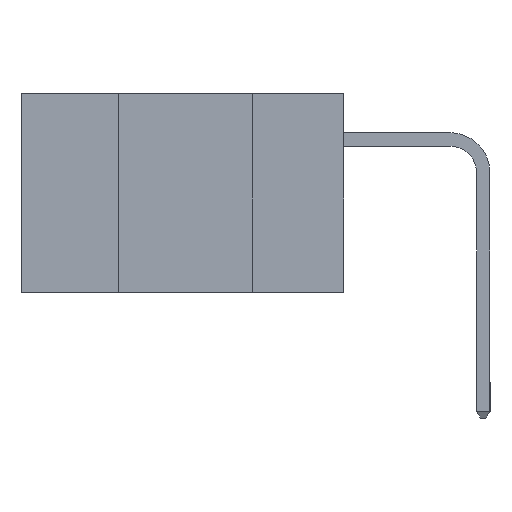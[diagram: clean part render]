
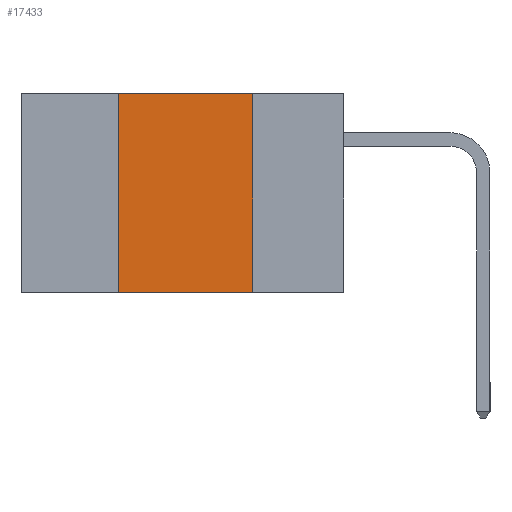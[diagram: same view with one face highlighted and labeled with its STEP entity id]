
A CAD part, left-side view. The second image highlights one B-rep face of the part: STEP entity #17433.
In plain terms, the highlighted planar face has unit normal (-1, 0, 0).
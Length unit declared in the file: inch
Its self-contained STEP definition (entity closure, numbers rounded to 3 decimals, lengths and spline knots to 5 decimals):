
#404 = DIRECTION ( 'NONE',  ( 0., -1., 0. ) ) ;
#518 = DIRECTION ( 'NONE',  ( 1., 0., 0. ) ) ;
#1114 = VECTOR ( 'NONE', #4299, 39.37008 ) ;
#1118 = EDGE_CURVE ( 'NONE', #13708, #14246, #14760, .T. ) ;
#1852 = VERTEX_POINT ( 'NONE', #10257 ) ;
#2001 = FACE_OUTER_BOUND ( 'NONE', #20241, .T. ) ;
#3552 = VECTOR ( 'NONE', #12343, 39.37008 ) ;
#4287 = EDGE_CURVE ( 'NONE', #6166, #1852, #16192, .T. ) ;
#4299 = DIRECTION ( 'NONE',  ( 0., -1., 0. ) ) ;
#4332 = CARTESIAN_POINT ( 'NONE',  ( 0., 0.42, 0. ) ) ;
#4366 = ORIENTED_EDGE ( 'NONE', *, *, #4287, .F. ) ;
#5296 = LINE ( 'NONE', #10690, #1114 ) ;
#5498 = EDGE_CURVE ( 'NONE', #14246, #6166, #17104, .T. ) ;
#6166 = VERTEX_POINT ( 'NONE', #7001 ) ;
#7001 = CARTESIAN_POINT ( 'NONE',  ( 0., 0.17, 0. ) ) ;
#7870 = ORIENTED_EDGE ( 'NONE', *, *, #1118, .F. ) ;
#8065 = ORIENTED_EDGE ( 'NONE', *, *, #5498, .F. ) ;
#8709 = VECTOR ( 'NONE', #404, 39.37008 ) ;
#9463 = ORIENTED_EDGE ( 'NONE', *, *, #19448, .T. ) ;
#9976 = PLANE ( 'NONE',  #12030 ) ;
#10257 = CARTESIAN_POINT ( 'NONE',  ( 0., 0.17, -0.37 ) ) ;
#10528 = VECTOR ( 'NONE', #14099, 39.37008 ) ;
#10690 = CARTESIAN_POINT ( 'NONE',  ( 0., 0.6, -0.37 ) ) ;
#11589 = DIRECTION ( 'NONE',  ( 0., 0., -1. ) ) ;
#12030 = AXIS2_PLACEMENT_3D ( 'NONE', #17803, #518, #11589 ) ;
#12343 = DIRECTION ( 'NONE',  ( 0., 0., -1. ) ) ;
#12582 = CARTESIAN_POINT ( 'NONE',  ( 0., 0.17, 0. ) ) ;
#13085 = CARTESIAN_POINT ( 'NONE',  ( 0., 0.6, 0. ) ) ;
#13708 = VERTEX_POINT ( 'NONE', #17598 ) ;
#14099 = DIRECTION ( 'NONE',  ( 0., 0., 1. ) ) ;
#14246 = VERTEX_POINT ( 'NONE', #15097 ) ;
#14760 = LINE ( 'NONE', #4332, #10528 ) ;
#15097 = CARTESIAN_POINT ( 'NONE',  ( 0., 0.42, 0. ) ) ;
#16192 = LINE ( 'NONE', #12582, #3552 ) ;
#17104 = LINE ( 'NONE', #13085, #8709 ) ;
#17433 = ADVANCED_FACE ( 'NONE', ( #2001 ), #9976, .F. ) ;
#17598 = CARTESIAN_POINT ( 'NONE',  ( 0., 0.42, -0.37 ) ) ;
#17803 = CARTESIAN_POINT ( 'NONE',  ( 0., 0.6, 0. ) ) ;
#19448 = EDGE_CURVE ( 'NONE', #13708, #1852, #5296, .T. ) ;
#20241 = EDGE_LOOP ( 'NONE', ( #4366, #8065, #7870, #9463 ) ) ;
